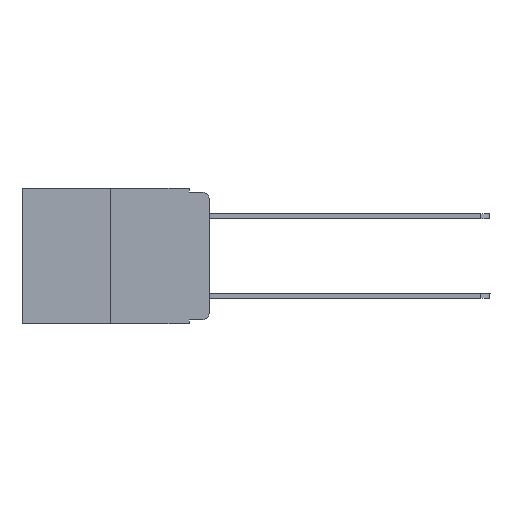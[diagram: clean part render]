
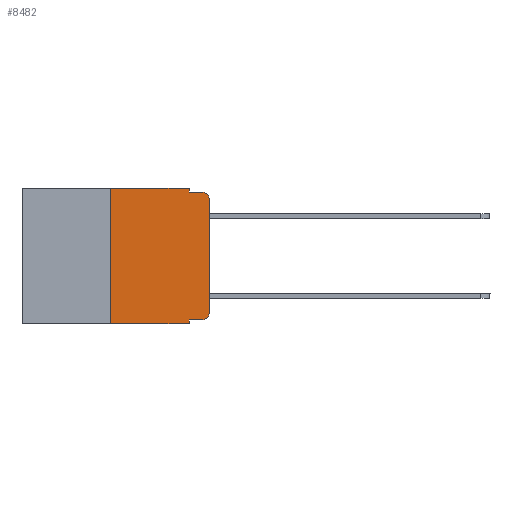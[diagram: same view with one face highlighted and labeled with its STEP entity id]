
A CAD part, left-side view. The second image highlights one B-rep face of the part: STEP entity #8482.
In plain terms, the highlighted planar face has unit normal (-1, 0, 0).
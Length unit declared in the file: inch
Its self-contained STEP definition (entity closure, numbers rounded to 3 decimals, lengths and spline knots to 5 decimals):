
#8 = FACE_OUTER_BOUND ( 'NONE', #15121, .T. ) ;
#594 = DIRECTION ( 'NONE',  ( 0., -1., 0. ) ) ;
#750 = EDGE_CURVE ( 'NONE', #4795, #5332, #14125, .T. ) ;
#1021 = CARTESIAN_POINT ( 'NONE',  ( 0., 0.02, -0.313 ) ) ;
#1149 = DIRECTION ( 'NONE',  ( 0., 0., -1. ) ) ;
#1339 = CARTESIAN_POINT ( 'NONE',  ( 0., 0.02, -0.333 ) ) ;
#1525 = EDGE_CURVE ( 'NONE', #10155, #14754, #11803, .T. ) ;
#1833 = CARTESIAN_POINT ( 'NONE',  ( 0., 0.051, -0.01 ) ) ;
#2024 = ORIENTED_EDGE ( 'NONE', *, *, #8859, .F. ) ;
#2519 = CIRCLE ( 'NONE', #4886, 0.02 ) ;
#2600 = ORIENTED_EDGE ( 'NONE', *, *, #9650, .T. ) ;
#2612 = VERTEX_POINT ( 'NONE', #12403 ) ;
#2616 = VECTOR ( 'NONE', #12259, 39.37008 ) ;
#2777 = CARTESIAN_POINT ( 'NONE',  ( 0., 0.051, -0.343 ) ) ;
#3323 = CARTESIAN_POINT ( 'NONE',  ( 0., 0.473, 0. ) ) ;
#3657 = DIRECTION ( 'NONE',  ( 0., 0., -1. ) ) ;
#3825 = CARTESIAN_POINT ( 'NONE',  ( 0., 0.051, 0. ) ) ;
#3848 = ORIENTED_EDGE ( 'NONE', *, *, #11861, .F. ) ;
#3926 = ORIENTED_EDGE ( 'NONE', *, *, #1525, .F. ) ;
#3975 = VERTEX_POINT ( 'NONE', #2777 ) ;
#4123 = VECTOR ( 'NONE', #6823, 39.37008 ) ;
#4149 = DIRECTION ( 'NONE',  ( 0., -1., 0. ) ) ;
#4311 = ORIENTED_EDGE ( 'NONE', *, *, #750, .T. ) ;
#4397 = ORIENTED_EDGE ( 'NONE', *, *, #7561, .F. ) ;
#4633 = AXIS2_PLACEMENT_3D ( 'NONE', #8899, #12498, #3657 ) ;
#4704 = CARTESIAN_POINT ( 'NONE',  ( 0., 0.25, -0.343 ) ) ;
#4795 = VERTEX_POINT ( 'NONE', #15330 ) ;
#4886 = AXIS2_PLACEMENT_3D ( 'NONE', #12889, #6568, #10312 ) ;
#4962 = VECTOR ( 'NONE', #4149, 39.37008 ) ;
#5332 = VERTEX_POINT ( 'NONE', #15557 ) ;
#5473 = CARTESIAN_POINT ( 'NONE',  ( 0., 0.25, 0. ) ) ;
#5855 = LINE ( 'NONE', #3323, #2616 ) ;
#6428 = CARTESIAN_POINT ( 'NONE',  ( 0., 0.473, -0.343 ) ) ;
#6568 = DIRECTION ( 'NONE',  ( -1., 0., 0. ) ) ;
#6719 = CIRCLE ( 'NONE', #14402, 0.02 ) ;
#6823 = DIRECTION ( 'NONE',  ( 0., 0., 1. ) ) ;
#7561 = EDGE_CURVE ( 'NONE', #2612, #12394, #9314, .T. ) ;
#7701 = CARTESIAN_POINT ( 'NONE',  ( 0., 0.051, 0. ) ) ;
#7839 = CARTESIAN_POINT ( 'NONE',  ( 0., 0., 0. ) ) ;
#8266 = ORIENTED_EDGE ( 'NONE', *, *, #9977, .T. ) ;
#8482 = ADVANCED_FACE ( 'NONE', ( #8 ), #11264, .F. ) ;
#8714 = CARTESIAN_POINT ( 'NONE',  ( 0., 0.051, 0. ) ) ;
#8859 = EDGE_CURVE ( 'NONE', #14112, #3975, #11065, .T. ) ;
#8899 = CARTESIAN_POINT ( 'NONE',  ( 0., 0.473, 0. ) ) ;
#9314 = LINE ( 'NONE', #1833, #10390 ) ;
#9650 = EDGE_CURVE ( 'NONE', #12062, #4795, #6719, .T. ) ;
#9735 = VECTOR ( 'NONE', #11066, 39.37008 ) ;
#9747 = DIRECTION ( 'NONE',  ( 0., 0., -1. ) ) ;
#9803 = CARTESIAN_POINT ( 'NONE',  ( 0., 0.02, -0.01 ) ) ;
#9926 = EDGE_CURVE ( 'NONE', #14314, #2612, #15112, .T. ) ;
#9977 = EDGE_CURVE ( 'NONE', #5332, #12394, #2519, .T. ) ;
#10155 = VERTEX_POINT ( 'NONE', #4704 ) ;
#10312 = DIRECTION ( 'NONE',  ( 0., 0., -1. ) ) ;
#10390 = VECTOR ( 'NONE', #594, 39.37008 ) ;
#10413 = LINE ( 'NONE', #6428, #4962 ) ;
#10555 = VECTOR ( 'NONE', #10606, 39.37008 ) ;
#10606 = DIRECTION ( 'NONE',  ( 0., 0., 1. ) ) ;
#10808 = ORIENTED_EDGE ( 'NONE', *, *, #14259, .T. ) ;
#10861 = DIRECTION ( 'NONE',  ( -1., 0., 0. ) ) ;
#10982 = LINE ( 'NONE', #12311, #9735 ) ;
#11065 = LINE ( 'NONE', #8714, #14913 ) ;
#11066 = DIRECTION ( 'NONE',  ( 0., -1., 0. ) ) ;
#11240 = VECTOR ( 'NONE', #13879, 39.37008 ) ;
#11264 = PLANE ( 'NONE',  #4633 ) ;
#11803 = LINE ( 'NONE', #5473, #10555 ) ;
#11861 = EDGE_CURVE ( 'NONE', #14754, #14314, #5855, .T. ) ;
#12062 = VERTEX_POINT ( 'NONE', #1339 ) ;
#12259 = DIRECTION ( 'NONE',  ( 0., -1., 0. ) ) ;
#12311 = CARTESIAN_POINT ( 'NONE',  ( 0., 0.051, -0.333 ) ) ;
#12394 = VERTEX_POINT ( 'NONE', #9803 ) ;
#12403 = CARTESIAN_POINT ( 'NONE',  ( 0., 0.051, -0.01 ) ) ;
#12498 = DIRECTION ( 'NONE',  ( 1., 0., 0. ) ) ;
#12889 = CARTESIAN_POINT ( 'NONE',  ( 0., 0.02, -0.03 ) ) ;
#13052 = EDGE_CURVE ( 'NONE', #10155, #3975, #10413, .T. ) ;
#13476 = ORIENTED_EDGE ( 'NONE', *, *, #13052, .T. ) ;
#13879 = DIRECTION ( 'NONE',  ( 0., 0., -1. ) ) ;
#13902 = CARTESIAN_POINT ( 'NONE',  ( 0., 0.25, 0. ) ) ;
#14112 = VERTEX_POINT ( 'NONE', #15579 ) ;
#14125 = LINE ( 'NONE', #7839, #4123 ) ;
#14259 = EDGE_CURVE ( 'NONE', #14112, #12062, #10982, .T. ) ;
#14314 = VERTEX_POINT ( 'NONE', #7701 ) ;
#14402 = AXIS2_PLACEMENT_3D ( 'NONE', #1021, #10861, #9747 ) ;
#14754 = VERTEX_POINT ( 'NONE', #13902 ) ;
#14913 = VECTOR ( 'NONE', #1149, 39.37008 ) ;
#15112 = LINE ( 'NONE', #3825, #11240 ) ;
#15121 = EDGE_LOOP ( 'NONE', ( #4311, #8266, #4397, #15742, #3848, #3926, #13476, #2024, #10808, #2600 ) ) ;
#15330 = CARTESIAN_POINT ( 'NONE',  ( 0., 0., -0.313 ) ) ;
#15557 = CARTESIAN_POINT ( 'NONE',  ( 0., 0., -0.03 ) ) ;
#15579 = CARTESIAN_POINT ( 'NONE',  ( 0., 0.051, -0.333 ) ) ;
#15742 = ORIENTED_EDGE ( 'NONE', *, *, #9926, .F. ) ;
